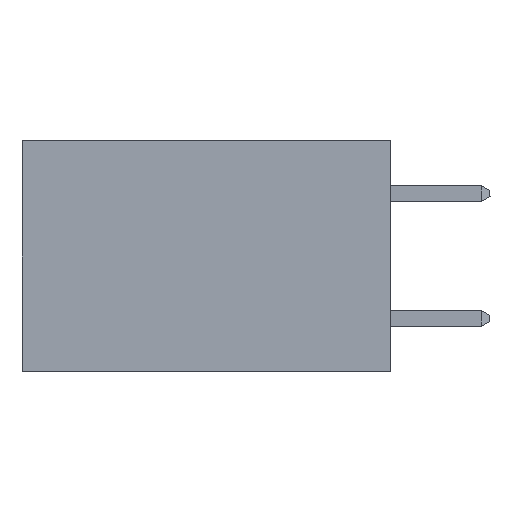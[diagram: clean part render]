
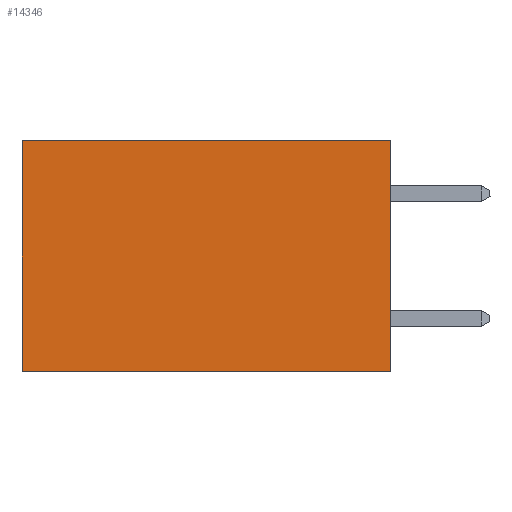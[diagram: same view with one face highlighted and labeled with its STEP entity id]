
A CAD part, left-side view. The second image highlights one B-rep face of the part: STEP entity #14346.
In plain terms, the highlighted planar face has unit normal (-1, 0, 0).
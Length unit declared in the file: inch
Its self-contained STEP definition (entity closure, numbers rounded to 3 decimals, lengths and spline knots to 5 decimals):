
#407 = DIRECTION ( 'NONE',  ( 0., 0., -1. ) ) ;
#899 = LINE ( 'NONE', #17965, #22789 ) ;
#912 = LINE ( 'NONE', #13700, #8237 ) ;
#1365 = VERTEX_POINT ( 'NONE', #14342 ) ;
#1502 = AXIS2_PLACEMENT_3D ( 'NONE', #27168, #18714, #5560 ) ;
#1997 = ORIENTED_EDGE ( 'NONE', *, *, #17803, .T. ) ;
#2276 = LINE ( 'NONE', #18702, #14764 ) ;
#4130 = EDGE_CURVE ( 'NONE', #22712, #20169, #899, .T. ) ;
#4768 = VERTEX_POINT ( 'NONE', #23286 ) ;
#5546 = DIRECTION ( 'NONE',  ( 0., 1., 0. ) ) ;
#5560 = DIRECTION ( 'NONE',  ( 0., 0., -1. ) ) ;
#7578 = VECTOR ( 'NONE', #22245, 39.37008 ) ;
#8237 = VECTOR ( 'NONE', #407, 39.37008 ) ;
#10989 = ORIENTED_EDGE ( 'NONE', *, *, #25571, .F. ) ;
#11119 = ORIENTED_EDGE ( 'NONE', *, *, #4130, .T. ) ;
#13446 = LINE ( 'NONE', #18021, #7578 ) ;
#13700 = CARTESIAN_POINT ( 'NONE',  ( 0.277, 0., -0.37 ) ) ;
#13800 = CARTESIAN_POINT ( 'NONE',  ( 0.277, 0.59, 0. ) ) ;
#14342 = CARTESIAN_POINT ( 'NONE',  ( 0.277, 0., 0. ) ) ;
#14346 = ADVANCED_FACE ( 'NONE', ( #16628 ), #22856, .F. ) ;
#14764 = VECTOR ( 'NONE', #5546, 39.37008 ) ;
#16628 = FACE_OUTER_BOUND ( 'NONE', #26423, .T. ) ;
#17386 = DIRECTION ( 'NONE',  ( 0., 0., -1. ) ) ;
#17803 = EDGE_CURVE ( 'NONE', #1365, #22712, #2276, .T. ) ;
#17965 = CARTESIAN_POINT ( 'NONE',  ( 0.277, 0.59, -0.37 ) ) ;
#18021 = CARTESIAN_POINT ( 'NONE',  ( 0.277, 0., -0.37 ) ) ;
#18264 = EDGE_CURVE ( 'NONE', #4768, #20169, #13446, .T. ) ;
#18295 = ORIENTED_EDGE ( 'NONE', *, *, #18264, .F. ) ;
#18702 = CARTESIAN_POINT ( 'NONE',  ( 0.277, 0., 0. ) ) ;
#18714 = DIRECTION ( 'NONE',  ( 1., 0., 0. ) ) ;
#20169 = VERTEX_POINT ( 'NONE', #26942 ) ;
#22245 = DIRECTION ( 'NONE',  ( 0., 1., 0. ) ) ;
#22712 = VERTEX_POINT ( 'NONE', #13800 ) ;
#22789 = VECTOR ( 'NONE', #17386, 39.37008 ) ;
#22856 = PLANE ( 'NONE',  #1502 ) ;
#23286 = CARTESIAN_POINT ( 'NONE',  ( 0.277, 0., -0.37 ) ) ;
#25571 = EDGE_CURVE ( 'NONE', #1365, #4768, #912, .T. ) ;
#26423 = EDGE_LOOP ( 'NONE', ( #11119, #18295, #10989, #1997 ) ) ;
#26942 = CARTESIAN_POINT ( 'NONE',  ( 0.277, 0.59, -0.37 ) ) ;
#27168 = CARTESIAN_POINT ( 'NONE',  ( 0.277, 0., -0.37 ) ) ;
